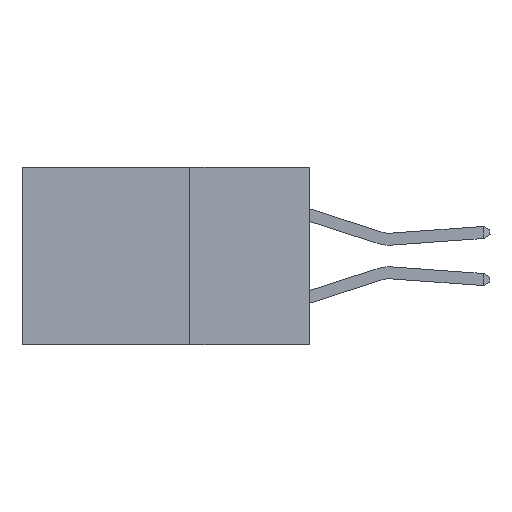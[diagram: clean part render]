
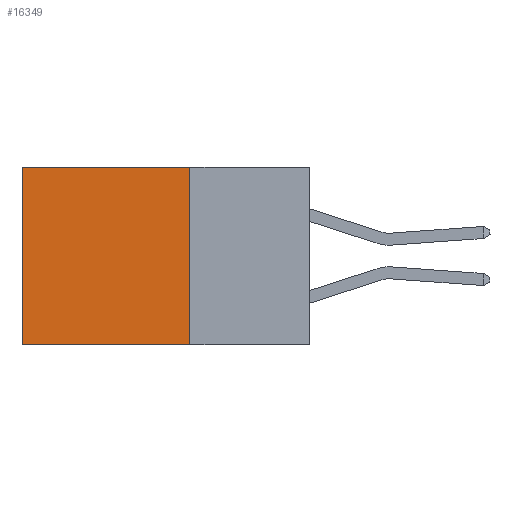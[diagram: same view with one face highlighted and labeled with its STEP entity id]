
A CAD part, left-side view. The second image highlights one B-rep face of the part: STEP entity #16349.
In plain terms, the highlighted planar face has unit normal (-1, 0, 0).
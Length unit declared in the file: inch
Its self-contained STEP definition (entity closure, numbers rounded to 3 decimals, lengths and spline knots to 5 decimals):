
#341 = CARTESIAN_POINT ( 'NONE',  ( 0.298, 0.25, 0. ) ) ;
#539 = CARTESIAN_POINT ( 'NONE',  ( 0.298, 0.25, -0.37 ) ) ;
#1089 = LINE ( 'NONE', #24407, #10846 ) ;
#1094 = EDGE_CURVE ( 'NONE', #12798, #20646, #19354, .T. ) ;
#3172 = DIRECTION ( 'NONE',  ( 1., 0., 0. ) ) ;
#4565 = VERTEX_POINT ( 'NONE', #539 ) ;
#5052 = EDGE_CURVE ( 'NONE', #19085, #4565, #18102, .T. ) ;
#6007 = DIRECTION ( 'NONE',  ( 0., 1., 0. ) ) ;
#7027 = CARTESIAN_POINT ( 'NONE',  ( 0.298, 0.25, 0. ) ) ;
#7254 = VECTOR ( 'NONE', #16930, 39.37008 ) ;
#7357 = VECTOR ( 'NONE', #6007, 39.37008 ) ;
#7538 = ORIENTED_EDGE ( 'NONE', *, *, #5052, .F. ) ;
#7963 = CARTESIAN_POINT ( 'NONE',  ( 0.298, 0.6, 0. ) ) ;
#8135 = EDGE_LOOP ( 'NONE', ( #17420, #17550, #7538, #23981 ) ) ;
#9274 = DIRECTION ( 'NONE',  ( 0., 1., 0. ) ) ;
#10846 = VECTOR ( 'NONE', #9274, 39.37008 ) ;
#11228 = CARTESIAN_POINT ( 'NONE',  ( 0.298, 0.6, -0.37 ) ) ;
#12798 = VERTEX_POINT ( 'NONE', #17216 ) ;
#14265 = VECTOR ( 'NONE', #17597, 39.37008 ) ;
#16349 = ADVANCED_FACE ( 'NONE', ( #17404 ), #18648, .F. ) ;
#16930 = DIRECTION ( 'NONE',  ( 0., 0., -1. ) ) ;
#17216 = CARTESIAN_POINT ( 'NONE',  ( 0.298, 0.6, 0. ) ) ;
#17404 = FACE_OUTER_BOUND ( 'NONE', #8135, .T. ) ;
#17420 = ORIENTED_EDGE ( 'NONE', *, *, #1094, .T. ) ;
#17550 = ORIENTED_EDGE ( 'NONE', *, *, #21798, .F. ) ;
#17576 = CARTESIAN_POINT ( 'NONE',  ( 0.298, 0.25, 0. ) ) ;
#17597 = DIRECTION ( 'NONE',  ( 0., 0., -1. ) ) ;
#18102 = LINE ( 'NONE', #19517, #7254 ) ;
#18648 = PLANE ( 'NONE',  #24647 ) ;
#18984 = EDGE_CURVE ( 'NONE', #19085, #12798, #22633, .T. ) ;
#19085 = VERTEX_POINT ( 'NONE', #341 ) ;
#19354 = LINE ( 'NONE', #7963, #14265 ) ;
#19517 = CARTESIAN_POINT ( 'NONE',  ( 0.298, 0.25, 0. ) ) ;
#20646 = VERTEX_POINT ( 'NONE', #11228 ) ;
#21798 = EDGE_CURVE ( 'NONE', #4565, #20646, #1089, .T. ) ;
#22439 = DIRECTION ( 'NONE',  ( 0., 0., -1. ) ) ;
#22633 = LINE ( 'NONE', #17576, #7357 ) ;
#23981 = ORIENTED_EDGE ( 'NONE', *, *, #18984, .T. ) ;
#24407 = CARTESIAN_POINT ( 'NONE',  ( 0.298, 0.25, -0.37 ) ) ;
#24647 = AXIS2_PLACEMENT_3D ( 'NONE', #7027, #3172, #22439 ) ;
